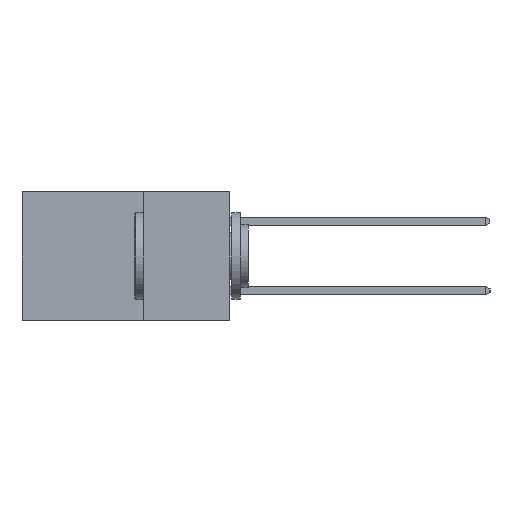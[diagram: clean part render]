
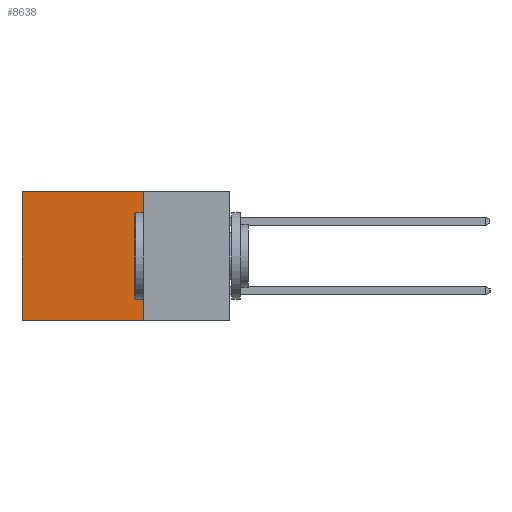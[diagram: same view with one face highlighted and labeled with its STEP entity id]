
A CAD part, left-side view. The second image highlights one B-rep face of the part: STEP entity #8638.
In plain terms, the highlighted planar face has unit normal (-1, 0, 0).
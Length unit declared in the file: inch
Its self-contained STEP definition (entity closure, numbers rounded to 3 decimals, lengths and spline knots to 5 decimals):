
#2582 = VECTOR ( 'NONE', #18943, 39.37008 ) ;
#2880 = EDGE_CURVE ( 'NONE', #18363, #20498, #19493, .T. ) ;
#4129 = AXIS2_PLACEMENT_3D ( 'NONE', #10992, #10365, #10339 ) ;
#4293 = CARTESIAN_POINT ( 'NONE',  ( 0.2615, 0.6, -0.37 ) ) ;
#4401 = EDGE_LOOP ( 'NONE', ( #11289, #16840, #14313, #20243 ) ) ;
#4616 = VERTEX_POINT ( 'NONE', #15466 ) ;
#5147 = VECTOR ( 'NONE', #8734, 39.37008 ) ;
#5703 = VERTEX_POINT ( 'NONE', #4293 ) ;
#5704 = CARTESIAN_POINT ( 'NONE',  ( 0.2615, 0.25, 0. ) ) ;
#5765 = VECTOR ( 'NONE', #13561, 39.37008 ) ;
#6345 = DIRECTION ( 'NONE',  ( 0., 0., -1. ) ) ;
#6869 = EDGE_CURVE ( 'NONE', #4616, #5703, #11925, .T. ) ;
#7076 = CARTESIAN_POINT ( 'NONE',  ( 0.2615, 0.25, 0. ) ) ;
#8120 = FACE_OUTER_BOUND ( 'NONE', #4401, .T. ) ;
#8638 = ADVANCED_FACE ( 'NONE', ( #8120 ), #11020, .F. ) ;
#8734 = DIRECTION ( 'NONE',  ( 0., 0., -1. ) ) ;
#9273 = LINE ( 'NONE', #20717, #5147 ) ;
#9480 = LINE ( 'NONE', #16632, #9714 ) ;
#9714 = VECTOR ( 'NONE', #6345, 39.37008 ) ;
#10339 = DIRECTION ( 'NONE',  ( 0., 0., -1. ) ) ;
#10365 = DIRECTION ( 'NONE',  ( 1., 0., 0. ) ) ;
#10992 = CARTESIAN_POINT ( 'NONE',  ( 0.2615, 0.25, -0.37 ) ) ;
#11020 = PLANE ( 'NONE',  #4129 ) ;
#11289 = ORIENTED_EDGE ( 'NONE', *, *, #14578, .T. ) ;
#11925 = LINE ( 'NONE', #22538, #2582 ) ;
#13561 = DIRECTION ( 'NONE',  ( 0., 1., 0. ) ) ;
#14313 = ORIENTED_EDGE ( 'NONE', *, *, #20891, .F. ) ;
#14578 = EDGE_CURVE ( 'NONE', #20498, #5703, #9480, .T. ) ;
#15466 = CARTESIAN_POINT ( 'NONE',  ( 0.2615, 0.25, -0.37 ) ) ;
#16286 = CARTESIAN_POINT ( 'NONE',  ( 0.2615, 0.6, 0. ) ) ;
#16632 = CARTESIAN_POINT ( 'NONE',  ( 0.2615, 0.6, -0.37 ) ) ;
#16840 = ORIENTED_EDGE ( 'NONE', *, *, #6869, .F. ) ;
#18363 = VERTEX_POINT ( 'NONE', #5704 ) ;
#18943 = DIRECTION ( 'NONE',  ( 0., 1., 0. ) ) ;
#19493 = LINE ( 'NONE', #7076, #5765 ) ;
#20243 = ORIENTED_EDGE ( 'NONE', *, *, #2880, .T. ) ;
#20498 = VERTEX_POINT ( 'NONE', #16286 ) ;
#20717 = CARTESIAN_POINT ( 'NONE',  ( 0.2615, 0.25, -0.37 ) ) ;
#20891 = EDGE_CURVE ( 'NONE', #18363, #4616, #9273, .T. ) ;
#22538 = CARTESIAN_POINT ( 'NONE',  ( 0.2615, 0.25, -0.37 ) ) ;
